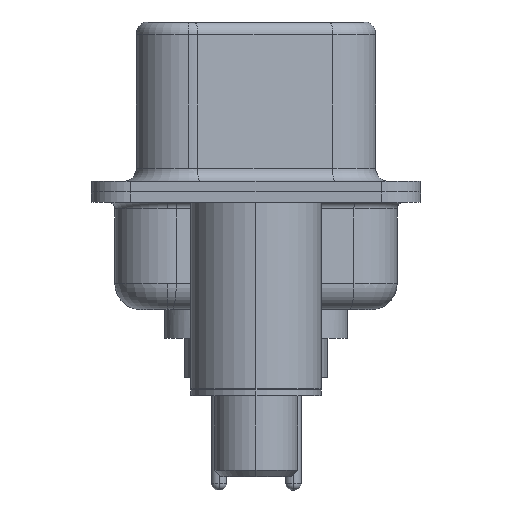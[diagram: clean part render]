
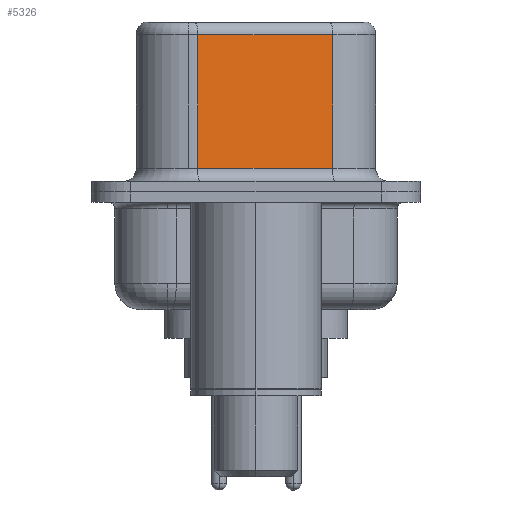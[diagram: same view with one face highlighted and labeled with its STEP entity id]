
A CAD part, left-side view. The second image highlights one B-rep face of the part: STEP entity #5326.
In plain terms, the highlighted planar face has unit normal (-0.985, -0.174, 0).
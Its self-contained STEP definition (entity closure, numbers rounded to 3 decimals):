
#492 = DIRECTION ( 'NONE',  ( 0.985, 0.174, 0. ) ) ;
#691 = ORIENTED_EDGE ( 'NONE', *, *, #10107, .T. ) ;
#747 = DIRECTION ( 'NONE',  ( 0.174, -0.985, 0. ) ) ;
#1593 = CARTESIAN_POINT ( 'NONE',  ( 4.585, -2.927, 6.02 ) ) ;
#1903 = CARTESIAN_POINT ( 'NONE',  ( 4.585, -2.927, 6.52 ) ) ;
#2055 = AXIS2_PLACEMENT_3D ( 'NONE', #1903, #492, #10628 ) ;
#2322 = CARTESIAN_POINT ( 'NONE',  ( 4.585, -2.927, 6.52 ) ) ;
#2590 = LINE ( 'NONE', #1593, #17246 ) ;
#3047 = DIRECTION ( 'NONE',  ( -0.174, 0.985, 0. ) ) ;
#4048 = CARTESIAN_POINT ( 'NONE',  ( 3.675, 2.233, 6.02 ) ) ;
#4184 = ORIENTED_EDGE ( 'NONE', *, *, #6342, .T. ) ;
#4185 = FACE_OUTER_BOUND ( 'NONE', #8599, .T. ) ;
#4963 = CARTESIAN_POINT ( 'NONE',  ( 4.585, -2.927, 6.02 ) ) ;
#5326 = ADVANCED_FACE ( 'NONE', ( #4185 ), #9167, .F. ) ;
#6183 = VERTEX_POINT ( 'NONE', #4048 ) ;
#6342 = EDGE_CURVE ( 'NONE', #17425, #6183, #2590, .T. ) ;
#6828 = VECTOR ( 'NONE', #14041, 1000. ) ;
#7207 = EDGE_CURVE ( 'NONE', #14557, #12653, #16800, .T. ) ;
#7817 = CARTESIAN_POINT ( 'NONE',  ( 3.675, 2.233, 0.9 ) ) ;
#7840 = DIRECTION ( 'NONE',  ( 0., 0., -1. ) ) ;
#8599 = EDGE_LOOP ( 'NONE', ( #16629, #4184, #691, #13621 ) ) ;
#9167 = PLANE ( 'NONE',  #2055 ) ;
#9764 = EDGE_CURVE ( 'NONE', #17425, #12653, #10687, .T. ) ;
#10107 = EDGE_CURVE ( 'NONE', #6183, #14557, #13437, .T. ) ;
#10628 = DIRECTION ( 'NONE',  ( -0.174, 0.985, 0. ) ) ;
#10687 = LINE ( 'NONE', #2322, #6828 ) ;
#11301 = CARTESIAN_POINT ( 'NONE',  ( 4.585, -2.927, 0.9 ) ) ;
#12653 = VERTEX_POINT ( 'NONE', #11301 ) ;
#13308 = VECTOR ( 'NONE', #747, 1000. ) ;
#13437 = LINE ( 'NONE', #15138, #16917 ) ;
#13621 = ORIENTED_EDGE ( 'NONE', *, *, #7207, .T. ) ;
#14041 = DIRECTION ( 'NONE',  ( 0., 0., -1. ) ) ;
#14557 = VERTEX_POINT ( 'NONE', #7817 ) ;
#15138 = CARTESIAN_POINT ( 'NONE',  ( 3.675, 2.233, 6.52 ) ) ;
#16629 = ORIENTED_EDGE ( 'NONE', *, *, #9764, .F. ) ;
#16800 = LINE ( 'NONE', #18264, #13308 ) ;
#16917 = VECTOR ( 'NONE', #7840, 1000. ) ;
#17246 = VECTOR ( 'NONE', #3047, 1000. ) ;
#17425 = VERTEX_POINT ( 'NONE', #4963 ) ;
#18264 = CARTESIAN_POINT ( 'NONE',  ( 4.585, -2.927, 0.9 ) ) ;
